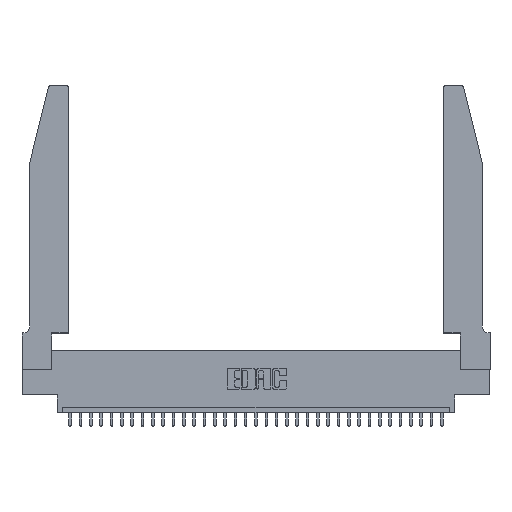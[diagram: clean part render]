
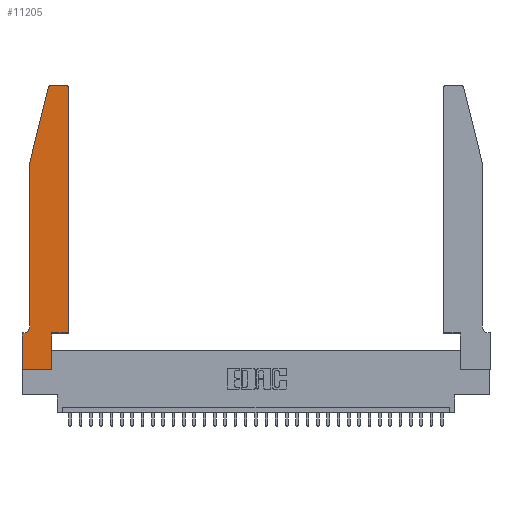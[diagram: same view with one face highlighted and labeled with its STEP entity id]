
A CAD part, top view. The second image highlights one B-rep face of the part: STEP entity #11205.
In plain terms, the highlighted planar face has unit normal (0, 0, 1).
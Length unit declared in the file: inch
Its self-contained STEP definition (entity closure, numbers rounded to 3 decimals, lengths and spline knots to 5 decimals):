
#1004 = VECTOR ( 'NONE', #13072, 39.37008 ) ;
#1119 = EDGE_CURVE ( 'NONE', #11697, #6372, #7336, .T. ) ;
#1131 = CARTESIAN_POINT ( 'NONE',  ( 0., 0.35, 0.37 ) ) ;
#1394 = CARTESIAN_POINT ( 'NONE',  ( 0.4205, 2.72, 0.37 ) ) ;
#1629 = ORIENTED_EDGE ( 'NONE', *, *, #9138, .T. ) ;
#2289 = VECTOR ( 'NONE', #5315, 39.37008 ) ;
#3089 = DIRECTION ( 'NONE',  ( 0., 1., 0. ) ) ;
#3178 = CIRCLE ( 'NONE', #32408, 0.03 ) ;
#3560 = DIRECTION ( 'NONE',  ( -1., 0., 0. ) ) ;
#3566 = LINE ( 'NONE', #13360, #29403 ) ;
#4659 = VECTOR ( 'NONE', #9603, 39.37008 ) ;
#4826 = CARTESIAN_POINT ( 'NONE',  ( 0.2605, 2.75, 0.37 ) ) ;
#5315 = DIRECTION ( 'NONE',  ( 1., 0., 0. ) ) ;
#5600 = ORIENTED_EDGE ( 'NONE', *, *, #23961, .T. ) ;
#6372 = VERTEX_POINT ( 'NONE', #27615 ) ;
#6479 = ORIENTED_EDGE ( 'NONE', *, *, #32527, .T. ) ;
#6603 = VERTEX_POINT ( 'NONE', #16400 ) ;
#7336 = LINE ( 'NONE', #18256, #30331 ) ;
#7750 = VERTEX_POINT ( 'NONE', #19327 ) ;
#8088 = DIRECTION ( 'NONE',  ( 0., 0., -1. ) ) ;
#8135 = CARTESIAN_POINT ( 'NONE',  ( 0., 0., 0.37 ) ) ;
#8428 = CARTESIAN_POINT ( 'NONE',  ( 0.0055, 0.42, 0.37 ) ) ;
#8581 = EDGE_CURVE ( 'NONE', #15200, #11188, #14769, .T. ) ;
#9109 = VECTOR ( 'NONE', #3089, 39.37008 ) ;
#9138 = EDGE_CURVE ( 'NONE', #16876, #11697, #15148, .T. ) ;
#9344 = LINE ( 'NONE', #26473, #11346 ) ;
#9603 = DIRECTION ( 'NONE',  ( -1., 0., 0. ) ) ;
#9682 = CARTESIAN_POINT ( 'NONE',  ( 0.2865, 0., 0.37 ) ) ;
#10922 = AXIS2_PLACEMENT_3D ( 'NONE', #15376, #28025, #15055 ) ;
#11113 = DIRECTION ( 'NONE',  ( 0., -1., 0. ) ) ;
#11188 = VERTEX_POINT ( 'NONE', #16105 ) ;
#11205 = ADVANCED_FACE ( 'NONE', ( #20304 ), #11372, .T. ) ;
#11346 = VECTOR ( 'NONE', #3560, 39.37008 ) ;
#11372 = PLANE ( 'NONE',  #20517 ) ;
#11697 = VERTEX_POINT ( 'NONE', #17594 ) ;
#11984 = VERTEX_POINT ( 'NONE', #14525 ) ;
#12416 = CARTESIAN_POINT ( 'NONE',  ( 0.0055, 0.35, 0.37 ) ) ;
#12658 = DIRECTION ( 'NONE',  ( -0.239, -0.971, 0. ) ) ;
#13060 = VERTEX_POINT ( 'NONE', #12416 ) ;
#13072 = DIRECTION ( 'NONE',  ( 0., 1., 0. ) ) ;
#13099 = ORIENTED_EDGE ( 'NONE', *, *, #22448, .T. ) ;
#13225 = LINE ( 'NONE', #20925, #18457 ) ;
#13360 = CARTESIAN_POINT ( 'NONE',  ( 0.0755, 2., 0.37 ) ) ;
#13816 = DIRECTION ( 'NONE',  ( 1., 0., 0. ) ) ;
#13836 = ORIENTED_EDGE ( 'NONE', *, *, #1119, .T. ) ;
#13963 = DIRECTION ( 'NONE',  ( 1., 0., 0. ) ) ;
#14008 = EDGE_CURVE ( 'NONE', #11188, #7750, #13225, .T. ) ;
#14267 = CARTESIAN_POINT ( 'NONE',  ( 0., 0., 0.37 ) ) ;
#14525 = CARTESIAN_POINT ( 'NONE',  ( 0.4505, 2.72, 0.37 ) ) ;
#14769 = CIRCLE ( 'NONE', #10922, 0.03 ) ;
#15055 = DIRECTION ( 'NONE',  ( 1., 0., 0. ) ) ;
#15148 = LINE ( 'NONE', #28824, #9109 ) ;
#15200 = VERTEX_POINT ( 'NONE', #20553 ) ;
#15376 = CARTESIAN_POINT ( 'NONE',  ( 0.284, 2.72, 0.37 ) ) ;
#15644 = LINE ( 'NONE', #15686, #2289 ) ;
#15686 = CARTESIAN_POINT ( 'NONE',  ( 0., 0., 0.37 ) ) ;
#16105 = CARTESIAN_POINT ( 'NONE',  ( 0.25487, 2.72718, 0.37 ) ) ;
#16400 = CARTESIAN_POINT ( 'NONE',  ( 0.4205, 2.75, 0.37 ) ) ;
#16876 = VERTEX_POINT ( 'NONE', #9682 ) ;
#17295 = EDGE_CURVE ( 'NONE', #22749, #29836, #20078, .T. ) ;
#17594 = CARTESIAN_POINT ( 'NONE',  ( 0.2865, 0.35, 0.37 ) ) ;
#18127 = EDGE_CURVE ( 'NONE', #6603, #15200, #28494, .T. ) ;
#18256 = CARTESIAN_POINT ( 'NONE',  ( 0.4505, 0.35, 0.37 ) ) ;
#18317 = EDGE_CURVE ( 'NONE', #6372, #11984, #32491, .T. ) ;
#18457 = VECTOR ( 'NONE', #12658, 39.37008 ) ;
#18604 = ORIENTED_EDGE ( 'NONE', *, *, #8581, .T. ) ;
#19117 = DIRECTION ( 'NONE',  ( 0., 0., 1. ) ) ;
#19327 = CARTESIAN_POINT ( 'NONE',  ( 0.0755, 2., 0.37 ) ) ;
#20064 = CIRCLE ( 'NONE', #33090, 0.07 ) ;
#20078 = LINE ( 'NONE', #14267, #32976 ) ;
#20304 = FACE_OUTER_BOUND ( 'NONE', #26996, .T. ) ;
#20517 = AXIS2_PLACEMENT_3D ( 'NONE', #29519, #31984, #13963 ) ;
#20553 = CARTESIAN_POINT ( 'NONE',  ( 0.284, 2.75, 0.37 ) ) ;
#20756 = DIRECTION ( 'NONE',  ( 1., 0., 0. ) ) ;
#20925 = CARTESIAN_POINT ( 'NONE',  ( 0.0755, 2., 0.37 ) ) ;
#21190 = DIRECTION ( 'NONE',  ( -1., 0., 0. ) ) ;
#21246 = ORIENTED_EDGE ( 'NONE', *, *, #18317, .T. ) ;
#22161 = ORIENTED_EDGE ( 'NONE', *, *, #31080, .T. ) ;
#22230 = VERTEX_POINT ( 'NONE', #26015 ) ;
#22448 = EDGE_CURVE ( 'NONE', #13060, #22749, #9344, .T. ) ;
#22749 = VERTEX_POINT ( 'NONE', #1131 ) ;
#23961 = EDGE_CURVE ( 'NONE', #7750, #22230, #3566, .T. ) ;
#24453 = EDGE_CURVE ( 'NONE', #29836, #16876, #15644, .T. ) ;
#26015 = CARTESIAN_POINT ( 'NONE',  ( 0.0755, 0.42, 0.37 ) ) ;
#26473 = CARTESIAN_POINT ( 'NONE',  ( 0.0755, 0.35, 0.37 ) ) ;
#26918 = DIRECTION ( 'NONE',  ( 0., -1., 0. ) ) ;
#26996 = EDGE_LOOP ( 'NONE', ( #27099, #18604, #28631, #5600, #6479, #13099, #27067, #27215, #1629, #13836, #21246, #22161 ) ) ;
#27067 = ORIENTED_EDGE ( 'NONE', *, *, #17295, .T. ) ;
#27099 = ORIENTED_EDGE ( 'NONE', *, *, #18127, .T. ) ;
#27215 = ORIENTED_EDGE ( 'NONE', *, *, #24453, .T. ) ;
#27615 = CARTESIAN_POINT ( 'NONE',  ( 0.4505, 0.35, 0.37 ) ) ;
#28025 = DIRECTION ( 'NONE',  ( 0., 0., 1. ) ) ;
#28494 = LINE ( 'NONE', #4826, #4659 ) ;
#28525 = CARTESIAN_POINT ( 'NONE',  ( 0.4505, 0.35, 0.37 ) ) ;
#28631 = ORIENTED_EDGE ( 'NONE', *, *, #14008, .T. ) ;
#28824 = CARTESIAN_POINT ( 'NONE',  ( 0.2865, 0.35, 0.37 ) ) ;
#29403 = VECTOR ( 'NONE', #11113, 39.37008 ) ;
#29519 = CARTESIAN_POINT ( 'NONE',  ( 0., 0.35, 0.37 ) ) ;
#29836 = VERTEX_POINT ( 'NONE', #8135 ) ;
#30331 = VECTOR ( 'NONE', #20756, 39.37008 ) ;
#31080 = EDGE_CURVE ( 'NONE', #11984, #6603, #3178, .T. ) ;
#31984 = DIRECTION ( 'NONE',  ( 0., 0., 1. ) ) ;
#32408 = AXIS2_PLACEMENT_3D ( 'NONE', #1394, #19117, #13816 ) ;
#32491 = LINE ( 'NONE', #28525, #1004 ) ;
#32527 = EDGE_CURVE ( 'NONE', #22230, #13060, #20064, .T. ) ;
#32976 = VECTOR ( 'NONE', #26918, 39.37008 ) ;
#33090 = AXIS2_PLACEMENT_3D ( 'NONE', #8428, #8088, #21190 ) ;
